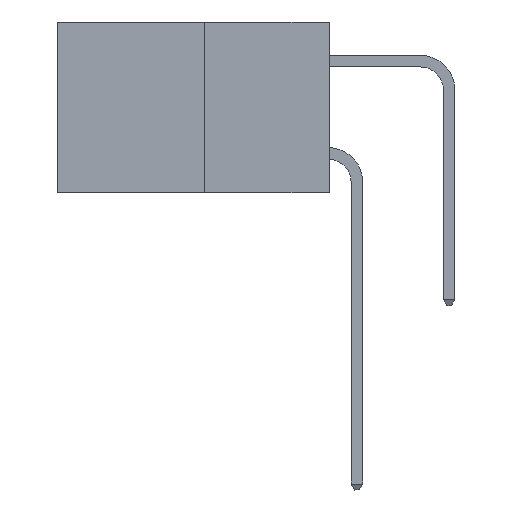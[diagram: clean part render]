
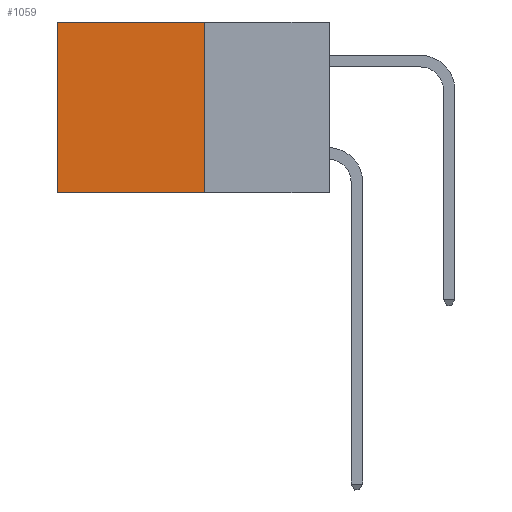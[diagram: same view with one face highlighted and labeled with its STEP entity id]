
A CAD part, left-side view. The second image highlights one B-rep face of the part: STEP entity #1059.
In plain terms, the highlighted planar face has unit normal (-1, 0, 0).
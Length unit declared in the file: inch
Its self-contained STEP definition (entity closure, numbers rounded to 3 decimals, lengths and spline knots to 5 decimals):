
#38 = VECTOR ( 'NONE', #9990, 39.37008 ) ;
#204 = VECTOR ( 'NONE', #6335, 39.37008 ) ;
#343 = LINE ( 'NONE', #7526, #10378 ) ;
#490 = AXIS2_PLACEMENT_3D ( 'NONE', #2011, #8601, #8577 ) ;
#1059 = ADVANCED_FACE ( 'NONE', ( #7980 ), #3293, .F. ) ;
#1566 = CARTESIAN_POINT ( 'NONE',  ( 0.277, 0.27, -0.37 ) ) ;
#1742 = VERTEX_POINT ( 'NONE', #8672 ) ;
#2011 = CARTESIAN_POINT ( 'NONE',  ( 0.277, 0.27, -0.37 ) ) ;
#2119 = ORIENTED_EDGE ( 'NONE', *, *, #5763, .F. ) ;
#2412 = DIRECTION ( 'NONE',  ( 0., 0., -1. ) ) ;
#2555 = DIRECTION ( 'NONE',  ( 0., 1., 0. ) ) ;
#3010 = EDGE_CURVE ( 'NONE', #7076, #3039, #4948, .T. ) ;
#3039 = VERTEX_POINT ( 'NONE', #9689 ) ;
#3293 = PLANE ( 'NONE',  #490 ) ;
#4588 = LINE ( 'NONE', #1566, #8572 ) ;
#4837 = LINE ( 'NONE', #5459, #204 ) ;
#4948 = LINE ( 'NONE', #10680, #38 ) ;
#5459 = CARTESIAN_POINT ( 'NONE',  ( 0.277, 0.27, 0. ) ) ;
#5763 = EDGE_CURVE ( 'NONE', #7594, #3039, #4588, .T. ) ;
#5996 = CARTESIAN_POINT ( 'NONE',  ( 0.277, 0.59, 0. ) ) ;
#6335 = DIRECTION ( 'NONE',  ( 0., 1., 0. ) ) ;
#6343 = EDGE_CURVE ( 'NONE', #1742, #7594, #343, .T. ) ;
#6389 = ORIENTED_EDGE ( 'NONE', *, *, #6533, .T. ) ;
#6533 = EDGE_CURVE ( 'NONE', #1742, #7076, #4837, .T. ) ;
#7076 = VERTEX_POINT ( 'NONE', #5996 ) ;
#7526 = CARTESIAN_POINT ( 'NONE',  ( 0.277, 0.27, -0.37 ) ) ;
#7594 = VERTEX_POINT ( 'NONE', #9297 ) ;
#7980 = FACE_OUTER_BOUND ( 'NONE', #10156, .T. ) ;
#8394 = ORIENTED_EDGE ( 'NONE', *, *, #3010, .T. ) ;
#8407 = ORIENTED_EDGE ( 'NONE', *, *, #6343, .F. ) ;
#8572 = VECTOR ( 'NONE', #2555, 39.37008 ) ;
#8577 = DIRECTION ( 'NONE',  ( 0., 0., -1. ) ) ;
#8601 = DIRECTION ( 'NONE',  ( 1., 0., 0. ) ) ;
#8672 = CARTESIAN_POINT ( 'NONE',  ( 0.277, 0.27, 0. ) ) ;
#9297 = CARTESIAN_POINT ( 'NONE',  ( 0.277, 0.27, -0.37 ) ) ;
#9689 = CARTESIAN_POINT ( 'NONE',  ( 0.277, 0.59, -0.37 ) ) ;
#9990 = DIRECTION ( 'NONE',  ( 0., 0., -1. ) ) ;
#10156 = EDGE_LOOP ( 'NONE', ( #8394, #2119, #8407, #6389 ) ) ;
#10378 = VECTOR ( 'NONE', #2412, 39.37008 ) ;
#10680 = CARTESIAN_POINT ( 'NONE',  ( 0.277, 0.59, -0.37 ) ) ;
